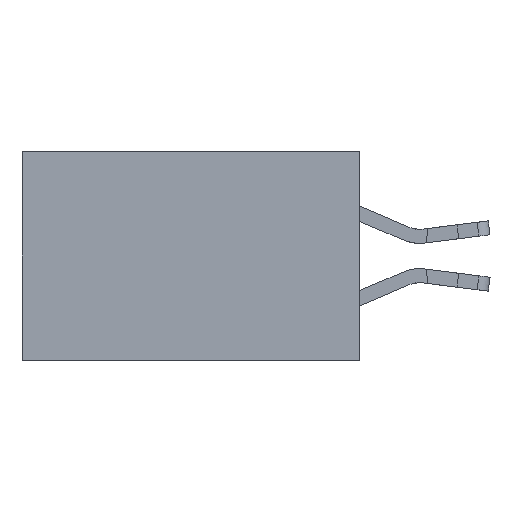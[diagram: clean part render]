
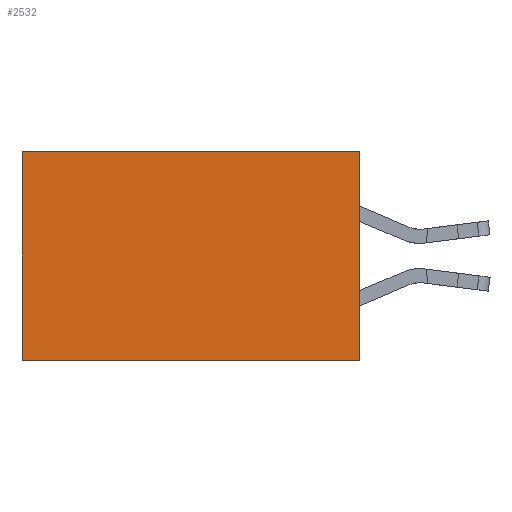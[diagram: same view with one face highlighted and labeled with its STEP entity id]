
A CAD part, left-side view. The second image highlights one B-rep face of the part: STEP entity #2532.
In plain terms, the highlighted planar face has unit normal (-1, 0, 0).
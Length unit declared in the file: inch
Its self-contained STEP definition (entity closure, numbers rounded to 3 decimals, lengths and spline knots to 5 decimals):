
#486 = VECTOR ( 'NONE', #10789, 39.37008 ) ;
#1228 = EDGE_CURVE ( 'NONE', #27414, #26079, #26569, .T. ) ;
#2532 = ADVANCED_FACE ( 'NONE', ( #10078 ), #17059, .F. ) ;
#3039 = VERTEX_POINT ( 'NONE', #23849 ) ;
#3766 = LINE ( 'NONE', #30045, #30560 ) ;
#3812 = AXIS2_PLACEMENT_3D ( 'NONE', #9872, #29420, #7425 ) ;
#3902 = CARTESIAN_POINT ( 'NONE',  ( 0.2875, 0., -0.37 ) ) ;
#5271 = CARTESIAN_POINT ( 'NONE',  ( 0.2875, 0., 0. ) ) ;
#5999 = CARTESIAN_POINT ( 'NONE',  ( 0.2875, 0., 0. ) ) ;
#6297 = VECTOR ( 'NONE', #16239, 39.37008 ) ;
#6454 = EDGE_CURVE ( 'NONE', #27414, #18547, #30025, .T. ) ;
#6867 = EDGE_LOOP ( 'NONE', ( #18200, #17126, #20741, #13630 ) ) ;
#7110 = VECTOR ( 'NONE', #25431, 39.37008 ) ;
#7425 = DIRECTION ( 'NONE',  ( 0., 0., -1. ) ) ;
#9872 = CARTESIAN_POINT ( 'NONE',  ( 0.2875, 0., 0. ) ) ;
#10078 = FACE_OUTER_BOUND ( 'NONE', #6867, .T. ) ;
#10789 = DIRECTION ( 'NONE',  ( 0., 0., -1. ) ) ;
#11052 = CARTESIAN_POINT ( 'NONE',  ( 0.2875, 0., 0. ) ) ;
#13630 = ORIENTED_EDGE ( 'NONE', *, *, #1228, .T. ) ;
#13983 = LINE ( 'NONE', #3902, #6297 ) ;
#16239 = DIRECTION ( 'NONE',  ( 0., 1., 0. ) ) ;
#17059 = PLANE ( 'NONE',  #3812 ) ;
#17126 = ORIENTED_EDGE ( 'NONE', *, *, #25076, .F. ) ;
#18200 = ORIENTED_EDGE ( 'NONE', *, *, #29737, .T. ) ;
#18547 = VERTEX_POINT ( 'NONE', #29644 ) ;
#20741 = ORIENTED_EDGE ( 'NONE', *, *, #6454, .F. ) ;
#23849 = CARTESIAN_POINT ( 'NONE',  ( 0.2875, 0.6, -0.37 ) ) ;
#25076 = EDGE_CURVE ( 'NONE', #18547, #3039, #13983, .T. ) ;
#25398 = DIRECTION ( 'NONE',  ( 0., 0., -1. ) ) ;
#25431 = DIRECTION ( 'NONE',  ( 0., 1., 0. ) ) ;
#26079 = VERTEX_POINT ( 'NONE', #27440 ) ;
#26569 = LINE ( 'NONE', #5999, #7110 ) ;
#27414 = VERTEX_POINT ( 'NONE', #11052 ) ;
#27440 = CARTESIAN_POINT ( 'NONE',  ( 0.2875, 0.6, 0. ) ) ;
#29420 = DIRECTION ( 'NONE',  ( 1., 0., 0. ) ) ;
#29644 = CARTESIAN_POINT ( 'NONE',  ( 0.2875, 0., -0.37 ) ) ;
#29737 = EDGE_CURVE ( 'NONE', #26079, #3039, #3766, .T. ) ;
#30025 = LINE ( 'NONE', #5271, #486 ) ;
#30045 = CARTESIAN_POINT ( 'NONE',  ( 0.2875, 0.6, 0. ) ) ;
#30560 = VECTOR ( 'NONE', #25398, 39.37008 ) ;
